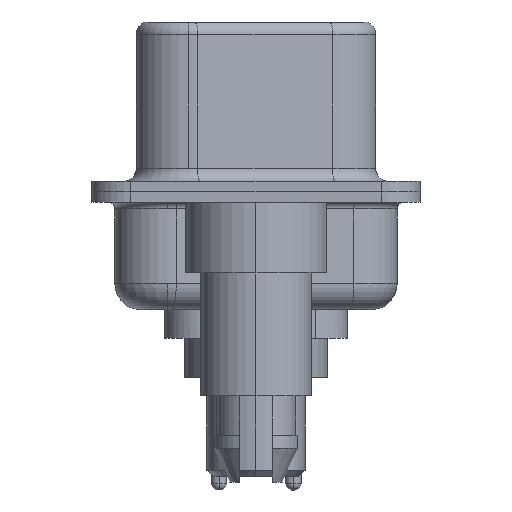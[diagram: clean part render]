
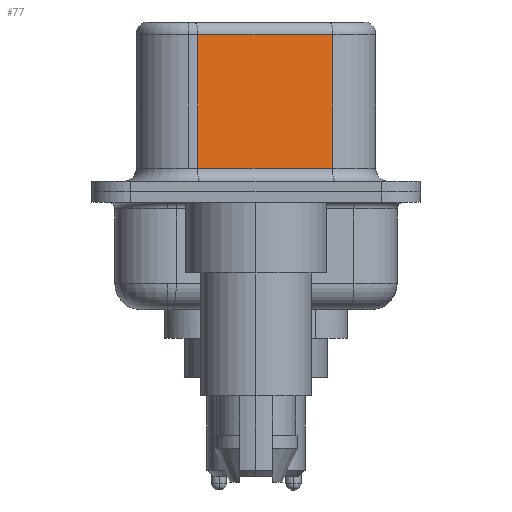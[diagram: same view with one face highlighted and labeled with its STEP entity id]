
A CAD part, left-side view. The second image highlights one B-rep face of the part: STEP entity #77.
In plain terms, the highlighted planar face has unit normal (-0.985, -0.174, 0).
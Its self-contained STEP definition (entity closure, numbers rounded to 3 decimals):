
#77 = ADVANCED_FACE ( 'NONE', ( #7309 ), #1320, .F. ) ;
#1320 = PLANE ( 'NONE',  #18707 ) ;
#2038 = VERTEX_POINT ( 'NONE', #12990 ) ;
#2716 = ORIENTED_EDGE ( 'NONE', *, *, #11961, .T. ) ;
#2733 = CARTESIAN_POINT ( 'NONE',  ( 4.585, -2.927, 6.02 ) ) ;
#4826 = CARTESIAN_POINT ( 'NONE',  ( 3.675, 2.233, 0.9 ) ) ;
#6343 = CARTESIAN_POINT ( 'NONE',  ( 4.585, -2.927, 0.9 ) ) ;
#6662 = VERTEX_POINT ( 'NONE', #4826 ) ;
#6758 = DIRECTION ( 'NONE',  ( 0., 0., -1. ) ) ;
#7142 = VERTEX_POINT ( 'NONE', #10932 ) ;
#7309 = FACE_OUTER_BOUND ( 'NONE', #16365, .T. ) ;
#7556 = LINE ( 'NONE', #18602, #14944 ) ;
#8674 = DIRECTION ( 'NONE',  ( -0.174, 0.985, 0. ) ) ;
#8699 = VECTOR ( 'NONE', #8674, 1000. ) ;
#8776 = EDGE_CURVE ( 'NONE', #9957, #2038, #11140, .T. ) ;
#9577 = CARTESIAN_POINT ( 'NONE',  ( 4.585, -2.927, 6.02 ) ) ;
#9957 = VERTEX_POINT ( 'NONE', #9577 ) ;
#10157 = CARTESIAN_POINT ( 'NONE',  ( 4.585, -2.927, 6.52 ) ) ;
#10416 = ORIENTED_EDGE ( 'NONE', *, *, #12628, .T. ) ;
#10932 = CARTESIAN_POINT ( 'NONE',  ( 3.675, 2.233, 6.02 ) ) ;
#11140 = LINE ( 'NONE', #13765, #18568 ) ;
#11961 = EDGE_CURVE ( 'NONE', #7142, #6662, #7556, .T. ) ;
#12264 = ORIENTED_EDGE ( 'NONE', *, *, #15213, .T. ) ;
#12628 = EDGE_CURVE ( 'NONE', #9957, #7142, #13065, .T. ) ;
#12990 = CARTESIAN_POINT ( 'NONE',  ( 4.585, -2.927, 0.9 ) ) ;
#13065 = LINE ( 'NONE', #2733, #8699 ) ;
#13179 = ORIENTED_EDGE ( 'NONE', *, *, #8776, .F. ) ;
#13765 = CARTESIAN_POINT ( 'NONE',  ( 4.585, -2.927, 6.52 ) ) ;
#13869 = LINE ( 'NONE', #6343, #14365 ) ;
#14365 = VECTOR ( 'NONE', #18179, 1000. ) ;
#14691 = DIRECTION ( 'NONE',  ( 0.985, 0.174, 0. ) ) ;
#14944 = VECTOR ( 'NONE', #6758, 1000. ) ;
#15213 = EDGE_CURVE ( 'NONE', #6662, #2038, #13869, .T. ) ;
#15570 = DIRECTION ( 'NONE',  ( -0.174, 0.985, 0. ) ) ;
#16365 = EDGE_LOOP ( 'NONE', ( #13179, #10416, #2716, #12264 ) ) ;
#18179 = DIRECTION ( 'NONE',  ( 0.174, -0.985, 0. ) ) ;
#18218 = DIRECTION ( 'NONE',  ( 0., 0., -1. ) ) ;
#18568 = VECTOR ( 'NONE', #18218, 1000. ) ;
#18602 = CARTESIAN_POINT ( 'NONE',  ( 3.675, 2.233, 6.52 ) ) ;
#18707 = AXIS2_PLACEMENT_3D ( 'NONE', #10157, #14691, #15570 ) ;
